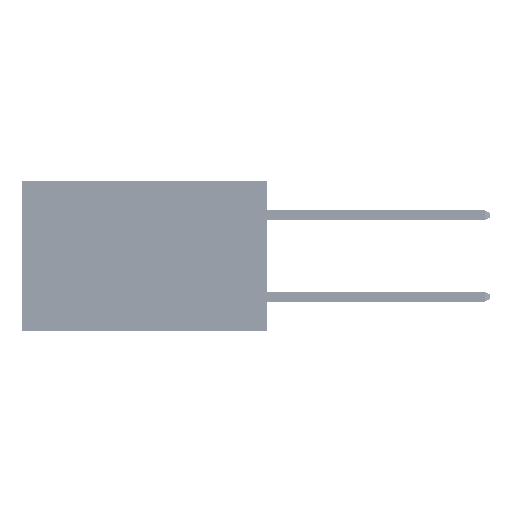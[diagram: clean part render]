
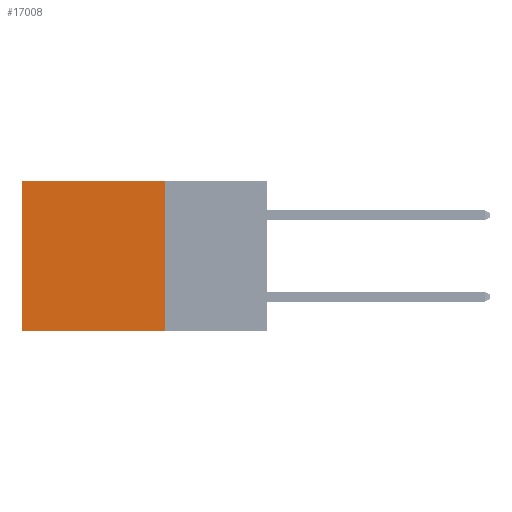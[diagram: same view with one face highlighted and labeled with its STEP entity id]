
A CAD part, left-side view. The second image highlights one B-rep face of the part: STEP entity #17008.
In plain terms, the highlighted planar face has unit normal (-1, 0, 0).
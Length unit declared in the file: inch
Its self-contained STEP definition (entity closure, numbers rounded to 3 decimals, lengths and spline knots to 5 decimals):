
#2755 = DIRECTION ( 'NONE',  ( 0., 0., -1. ) ) ;
#4209 = VERTEX_POINT ( 'NONE', #20477 ) ;
#5612 = EDGE_CURVE ( 'NONE', #40166, #10197, #42972, .T. ) ;
#5624 = CARTESIAN_POINT ( 'NONE',  ( 0.2875, 0.25, 0. ) ) ;
#7643 = VECTOR ( 'NONE', #38744, 39.37008 ) ;
#8353 = CARTESIAN_POINT ( 'NONE',  ( 0.2875, 0.6, 0. ) ) ;
#9609 = CARTESIAN_POINT ( 'NONE',  ( 0.2875, 0.25, -0.37 ) ) ;
#9778 = DIRECTION ( 'NONE',  ( 0., 1., 0. ) ) ;
#10197 = VERTEX_POINT ( 'NONE', #11344 ) ;
#11344 = CARTESIAN_POINT ( 'NONE',  ( 0.2875, 0.6, 0. ) ) ;
#12481 = CARTESIAN_POINT ( 'NONE',  ( 0.2875, 0.25, 0. ) ) ;
#14196 = VERTEX_POINT ( 'NONE', #42939 ) ;
#16636 = EDGE_CURVE ( 'NONE', #10197, #4209, #17772, .T. ) ;
#17008 = ADVANCED_FACE ( 'NONE', ( #36122 ), #48177, .F. ) ;
#17163 = DIRECTION ( 'NONE',  ( 0., 1., 0. ) ) ;
#17490 = LINE ( 'NONE', #9609, #36492 ) ;
#17772 = LINE ( 'NONE', #8353, #7643 ) ;
#20477 = CARTESIAN_POINT ( 'NONE',  ( 0.2875, 0.6, -0.37 ) ) ;
#23875 = CARTESIAN_POINT ( 'NONE',  ( 0.2875, 0.25, 0. ) ) ;
#25654 = DIRECTION ( 'NONE',  ( 1., 0., 0. ) ) ;
#28518 = VECTOR ( 'NONE', #39017, 39.37008 ) ;
#31504 = ORIENTED_EDGE ( 'NONE', *, *, #39103, .F. ) ;
#32988 = VECTOR ( 'NONE', #17163, 39.37008 ) ;
#33373 = ORIENTED_EDGE ( 'NONE', *, *, #16636, .T. ) ;
#33567 = EDGE_CURVE ( 'NONE', #40166, #14196, #37358, .T. ) ;
#35113 = ORIENTED_EDGE ( 'NONE', *, *, #5612, .T. ) ;
#35745 = AXIS2_PLACEMENT_3D ( 'NONE', #40648, #25654, #2755 ) ;
#36122 = FACE_OUTER_BOUND ( 'NONE', #42929, .T. ) ;
#36492 = VECTOR ( 'NONE', #9778, 39.37008 ) ;
#37358 = LINE ( 'NONE', #12481, #28518 ) ;
#38744 = DIRECTION ( 'NONE',  ( 0., 0., -1. ) ) ;
#39017 = DIRECTION ( 'NONE',  ( 0., 0., -1. ) ) ;
#39103 = EDGE_CURVE ( 'NONE', #14196, #4209, #17490, .T. ) ;
#40166 = VERTEX_POINT ( 'NONE', #23875 ) ;
#40648 = CARTESIAN_POINT ( 'NONE',  ( 0.2875, 0.25, 0. ) ) ;
#42501 = ORIENTED_EDGE ( 'NONE', *, *, #33567, .F. ) ;
#42929 = EDGE_LOOP ( 'NONE', ( #33373, #31504, #42501, #35113 ) ) ;
#42939 = CARTESIAN_POINT ( 'NONE',  ( 0.2875, 0.25, -0.37 ) ) ;
#42972 = LINE ( 'NONE', #5624, #32988 ) ;
#48177 = PLANE ( 'NONE',  #35745 ) ;
